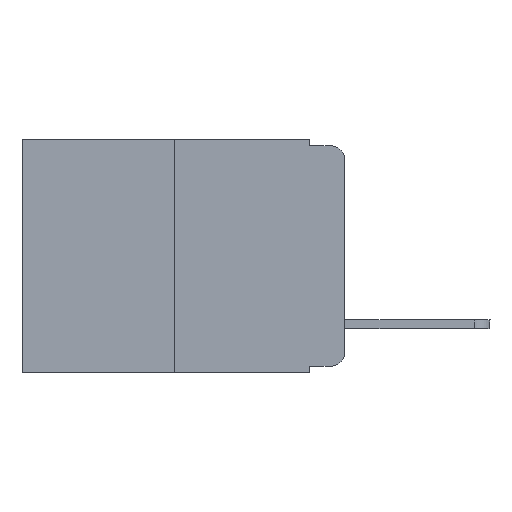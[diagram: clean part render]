
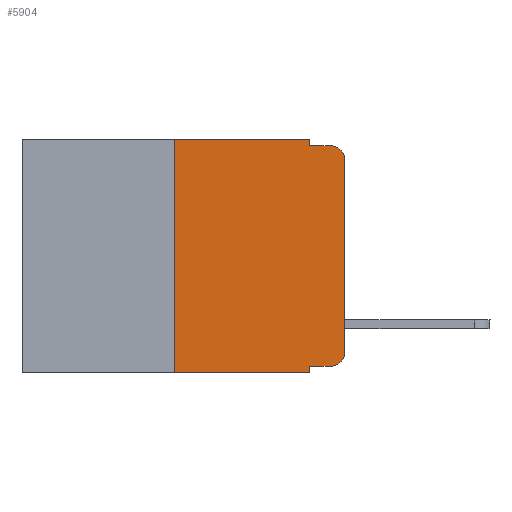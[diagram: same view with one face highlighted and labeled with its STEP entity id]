
A CAD part, left-side view. The second image highlights one B-rep face of the part: STEP entity #5904.
In plain terms, the highlighted planar face has unit normal (-1, 0, 0).
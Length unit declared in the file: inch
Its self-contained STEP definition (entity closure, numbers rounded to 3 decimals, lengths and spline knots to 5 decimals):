
#211 = CARTESIAN_POINT ( 'NONE',  ( 0., 0.051, 0. ) ) ;
#392 = DIRECTION ( 'NONE',  ( 0., -1., 0. ) ) ;
#620 = AXIS2_PLACEMENT_3D ( 'NONE', #22301, #10140, #16803 ) ;
#622 = ORIENTED_EDGE ( 'NONE', *, *, #1268, .F. ) ;
#723 = CARTESIAN_POINT ( 'NONE',  ( 0., 0.25, 0. ) ) ;
#737 = FACE_OUTER_BOUND ( 'NONE', #2948, .T. ) ;
#819 = AXIS2_PLACEMENT_3D ( 'NONE', #13934, #13584, #16921 ) ;
#965 = AXIS2_PLACEMENT_3D ( 'NONE', #13041, #20043, #9155 ) ;
#1086 = CARTESIAN_POINT ( 'NONE',  ( 0., 0.051, 0. ) ) ;
#1268 = EDGE_CURVE ( 'NONE', #8741, #15688, #9103, .T. ) ;
#1272 = VERTEX_POINT ( 'NONE', #11054 ) ;
#1310 = ORIENTED_EDGE ( 'NONE', *, *, #5103, .T. ) ;
#1330 = EDGE_CURVE ( 'NONE', #9986, #8361, #17826, .T. ) ;
#1665 = CARTESIAN_POINT ( 'NONE',  ( 0., 0.25, 0. ) ) ;
#2470 = VECTOR ( 'NONE', #8867, 39.37008 ) ;
#2832 = DIRECTION ( 'NONE',  ( 0., -1., 0. ) ) ;
#2948 = EDGE_LOOP ( 'NONE', ( #10322, #9640, #20446, #19707, #22089, #17335, #11120, #622, #1310, #15863 ) ) ;
#2987 = EDGE_CURVE ( 'NONE', #22114, #8188, #12560, .T. ) ;
#3809 = DIRECTION ( 'NONE',  ( 0., 0., 1. ) ) ;
#4457 = VERTEX_POINT ( 'NONE', #9985 ) ;
#5083 = CARTESIAN_POINT ( 'NONE',  ( 0., 0.02, -0.333 ) ) ;
#5103 = EDGE_CURVE ( 'NONE', #8741, #14680, #8005, .T. ) ;
#5109 = CARTESIAN_POINT ( 'NONE',  ( 0., 0.051, -0.343 ) ) ;
#5180 = EDGE_CURVE ( 'NONE', #5349, #9986, #19387, .T. ) ;
#5349 = VERTEX_POINT ( 'NONE', #11018 ) ;
#5394 = VECTOR ( 'NONE', #392, 39.37008 ) ;
#5644 = CARTESIAN_POINT ( 'NONE',  ( 0., 0., 0. ) ) ;
#5904 = ADVANCED_FACE ( 'NONE', ( #737 ), #6025, .F. ) ;
#6025 = PLANE ( 'NONE',  #965 ) ;
#6148 = CARTESIAN_POINT ( 'NONE',  ( 0., 0.473, -0.343 ) ) ;
#6274 = CARTESIAN_POINT ( 'NONE',  ( 0., 0.051, -0.333 ) ) ;
#6705 = EDGE_CURVE ( 'NONE', #14680, #22114, #16789, .T. ) ;
#6815 = EDGE_CURVE ( 'NONE', #1272, #4457, #12315, .T. ) ;
#6991 = VECTOR ( 'NONE', #7548, 39.37008 ) ;
#7548 = DIRECTION ( 'NONE',  ( 0., 0., -1. ) ) ;
#7662 = LINE ( 'NONE', #16297, #6991 ) ;
#8005 = LINE ( 'NONE', #6274, #22472 ) ;
#8188 = VERTEX_POINT ( 'NONE', #9271 ) ;
#8361 = VERTEX_POINT ( 'NONE', #1086 ) ;
#8601 = VECTOR ( 'NONE', #16114, 39.37008 ) ;
#8687 = DIRECTION ( 'NONE',  ( 0., 0., 1. ) ) ;
#8741 = VERTEX_POINT ( 'NONE', #13131 ) ;
#8867 = DIRECTION ( 'NONE',  ( 0., -1., 0. ) ) ;
#8942 = VECTOR ( 'NONE', #17939, 39.37008 ) ;
#8994 = CARTESIAN_POINT ( 'NONE',  ( 0., 0.051, -0.01 ) ) ;
#9103 = LINE ( 'NONE', #211, #8942 ) ;
#9155 = DIRECTION ( 'NONE',  ( 0., 0., -1. ) ) ;
#9271 = CARTESIAN_POINT ( 'NONE',  ( 0., 0., -0.03 ) ) ;
#9640 = ORIENTED_EDGE ( 'NONE', *, *, #10125, .T. ) ;
#9985 = CARTESIAN_POINT ( 'NONE',  ( 0., 0.02, -0.01 ) ) ;
#9986 = VERTEX_POINT ( 'NONE', #723 ) ;
#10125 = EDGE_CURVE ( 'NONE', #8188, #4457, #14779, .T. ) ;
#10140 = DIRECTION ( 'NONE',  ( -1., 0., 0. ) ) ;
#10322 = ORIENTED_EDGE ( 'NONE', *, *, #2987, .T. ) ;
#11018 = CARTESIAN_POINT ( 'NONE',  ( 0., 0.25, -0.343 ) ) ;
#11054 = CARTESIAN_POINT ( 'NONE',  ( 0., 0.051, -0.01 ) ) ;
#11120 = ORIENTED_EDGE ( 'NONE', *, *, #18475, .T. ) ;
#11244 = EDGE_CURVE ( 'NONE', #8361, #1272, #7662, .T. ) ;
#12315 = LINE ( 'NONE', #8994, #2470 ) ;
#12560 = LINE ( 'NONE', #5644, #13575 ) ;
#12783 = CARTESIAN_POINT ( 'NONE',  ( 0., 0., -0.313 ) ) ;
#13041 = CARTESIAN_POINT ( 'NONE',  ( 0., 0.473, 0. ) ) ;
#13131 = CARTESIAN_POINT ( 'NONE',  ( 0., 0.051, -0.333 ) ) ;
#13163 = LINE ( 'NONE', #6148, #5394 ) ;
#13575 = VECTOR ( 'NONE', #3809, 39.37008 ) ;
#13584 = DIRECTION ( 'NONE',  ( -1., 0., 0. ) ) ;
#13934 = CARTESIAN_POINT ( 'NONE',  ( 0., 0.02, -0.03 ) ) ;
#14680 = VERTEX_POINT ( 'NONE', #5083 ) ;
#14779 = CIRCLE ( 'NONE', #819, 0.02 ) ;
#15688 = VERTEX_POINT ( 'NONE', #5109 ) ;
#15863 = ORIENTED_EDGE ( 'NONE', *, *, #6705, .T. ) ;
#16114 = DIRECTION ( 'NONE',  ( 0., -1., 0. ) ) ;
#16223 = CARTESIAN_POINT ( 'NONE',  ( 0., 0.473, 0. ) ) ;
#16297 = CARTESIAN_POINT ( 'NONE',  ( 0., 0.051, 0. ) ) ;
#16789 = CIRCLE ( 'NONE', #620, 0.02 ) ;
#16803 = DIRECTION ( 'NONE',  ( 0., 0., -1. ) ) ;
#16921 = DIRECTION ( 'NONE',  ( 0., 0., -1. ) ) ;
#17335 = ORIENTED_EDGE ( 'NONE', *, *, #5180, .F. ) ;
#17826 = LINE ( 'NONE', #16223, #8601 ) ;
#17939 = DIRECTION ( 'NONE',  ( 0., 0., -1. ) ) ;
#18111 = VECTOR ( 'NONE', #8687, 39.37008 ) ;
#18475 = EDGE_CURVE ( 'NONE', #5349, #15688, #13163, .T. ) ;
#19387 = LINE ( 'NONE', #1665, #18111 ) ;
#19707 = ORIENTED_EDGE ( 'NONE', *, *, #11244, .F. ) ;
#20043 = DIRECTION ( 'NONE',  ( 1., 0., 0. ) ) ;
#20446 = ORIENTED_EDGE ( 'NONE', *, *, #6815, .F. ) ;
#22089 = ORIENTED_EDGE ( 'NONE', *, *, #1330, .F. ) ;
#22114 = VERTEX_POINT ( 'NONE', #12783 ) ;
#22301 = CARTESIAN_POINT ( 'NONE',  ( 0., 0.02, -0.313 ) ) ;
#22472 = VECTOR ( 'NONE', #2832, 39.37008 ) ;
